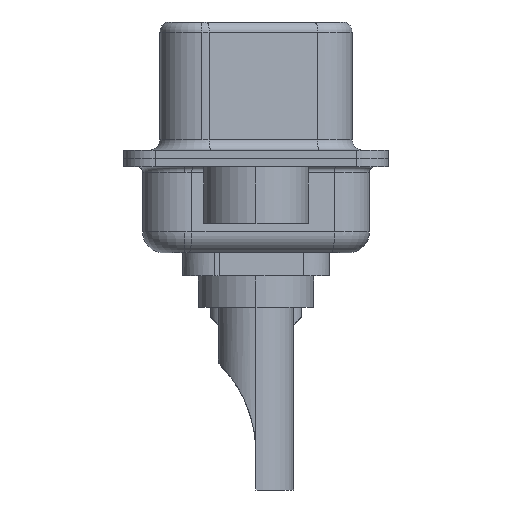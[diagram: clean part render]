
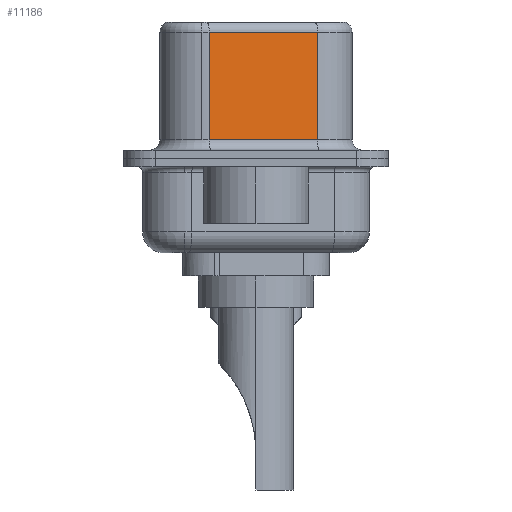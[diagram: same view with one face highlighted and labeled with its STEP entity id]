
A CAD part, left-side view. The second image highlights one B-rep face of the part: STEP entity #11186.
In plain terms, the highlighted planar face has unit normal (-0.985, -0.174, 0).
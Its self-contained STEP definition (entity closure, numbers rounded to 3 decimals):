
#189 = VECTOR ( 'NONE', #2053, 1000. ) ;
#1092 = CARTESIAN_POINT ( 'NONE',  ( 4.585, -2.927, 6.02 ) ) ;
#2053 = DIRECTION ( 'NONE',  ( 0., 0., -1. ) ) ;
#2261 = CARTESIAN_POINT ( 'NONE',  ( 4.585, -2.927, 6.02 ) ) ;
#2626 = CARTESIAN_POINT ( 'NONE',  ( 4.585, -2.927, 0.9 ) ) ;
#2762 = VECTOR ( 'NONE', #6757, 1000. ) ;
#3194 = FACE_OUTER_BOUND ( 'NONE', #12101, .T. ) ;
#3356 = VERTEX_POINT ( 'NONE', #15310 ) ;
#3992 = VERTEX_POINT ( 'NONE', #1092 ) ;
#4041 = CARTESIAN_POINT ( 'NONE',  ( 3.675, 2.233, 6.02 ) ) ;
#4254 = LINE ( 'NONE', #17440, #8663 ) ;
#4307 = ORIENTED_EDGE ( 'NONE', *, *, #8930, .F. ) ;
#5267 = VECTOR ( 'NONE', #10483, 1000. ) ;
#5667 = ORIENTED_EDGE ( 'NONE', *, *, #7829, .T. ) ;
#6757 = DIRECTION ( 'NONE',  ( 0.174, -0.985, 0. ) ) ;
#7165 = CARTESIAN_POINT ( 'NONE',  ( 4.585, -2.927, 0.9 ) ) ;
#7524 = PLANE ( 'NONE',  #16211 ) ;
#7829 = EDGE_CURVE ( 'NONE', #3356, #14610, #16034, .T. ) ;
#8663 = VECTOR ( 'NONE', #19055, 1000. ) ;
#8930 = EDGE_CURVE ( 'NONE', #3992, #14610, #4254, .T. ) ;
#10483 = DIRECTION ( 'NONE',  ( -0.174, 0.985, 0. ) ) ;
#10837 = DIRECTION ( 'NONE',  ( -0.174, 0.985, 0. ) ) ;
#11048 = EDGE_CURVE ( 'NONE', #3992, #21254, #17940, .T. ) ;
#11186 = ADVANCED_FACE ( 'NONE', ( #3194 ), #7524, .F. ) ;
#11189 = ORIENTED_EDGE ( 'NONE', *, *, #14399, .T. ) ;
#12101 = EDGE_LOOP ( 'NONE', ( #4307, #13289, #11189, #5667 ) ) ;
#13289 = ORIENTED_EDGE ( 'NONE', *, *, #11048, .T. ) ;
#13738 = CARTESIAN_POINT ( 'NONE',  ( 3.675, 2.233, 6.52 ) ) ;
#14399 = EDGE_CURVE ( 'NONE', #21254, #3356, #18324, .T. ) ;
#14610 = VERTEX_POINT ( 'NONE', #2626 ) ;
#15310 = CARTESIAN_POINT ( 'NONE',  ( 3.675, 2.233, 0.9 ) ) ;
#16034 = LINE ( 'NONE', #7165, #2762 ) ;
#16211 = AXIS2_PLACEMENT_3D ( 'NONE', #19081, #20713, #10837 ) ;
#17440 = CARTESIAN_POINT ( 'NONE',  ( 4.585, -2.927, 6.52 ) ) ;
#17940 = LINE ( 'NONE', #2261, #5267 ) ;
#18324 = LINE ( 'NONE', #13738, #189 ) ;
#19055 = DIRECTION ( 'NONE',  ( 0., 0., -1. ) ) ;
#19081 = CARTESIAN_POINT ( 'NONE',  ( 4.585, -2.927, 6.52 ) ) ;
#20713 = DIRECTION ( 'NONE',  ( 0.985, 0.174, 0. ) ) ;
#21254 = VERTEX_POINT ( 'NONE', #4041 ) ;
